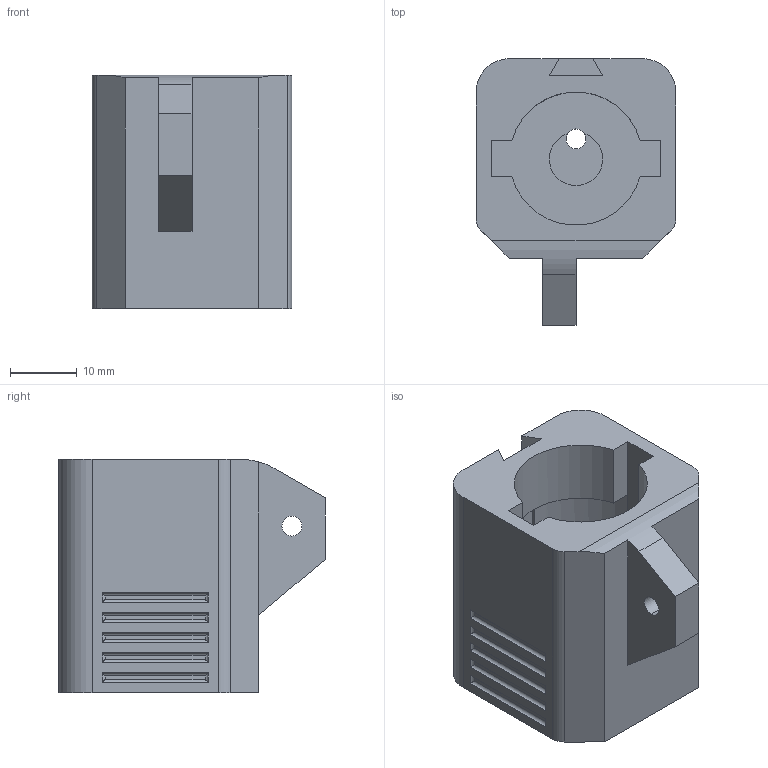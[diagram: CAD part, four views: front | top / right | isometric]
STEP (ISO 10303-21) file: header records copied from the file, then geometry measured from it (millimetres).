
FILE_DESCRIPTION (( 'STEP AP214' ), '1' );
FILE_NAME ('Receiver^StikM1.STEP', '2013-09-01T22:37:56', ( 'Asher' ), ( '' ), 'SwSTEP 2.0', 'SolidWorks 2013', '' );
FILE_SCHEMA (( 'AUTOMOTIVE_DESIGN' ));
Length unit declared in the file: millimetre
Products named in the file (1): Receiver^StikM1
Bounding box: 30 x 40 x 35 mm (x, y, z)
Volume: 19976.2 mm3; surface area: 8604.5 mm2
Topology: 1 solids, 1 shells, 241 faces, 645 edges, 428 vertices
Faces by surface type: plane 117, bspline 64, cylinder 58, cone 2
Entity records: 10656 total; most frequent: CARTESIAN_POINT 5105, ORIENTED_EDGE 1290, DIRECTION 874, EDGE_CURVE 645, LINE 432, VECTOR 432, VERTEX_POINT 428, EDGE_LOOP 269
